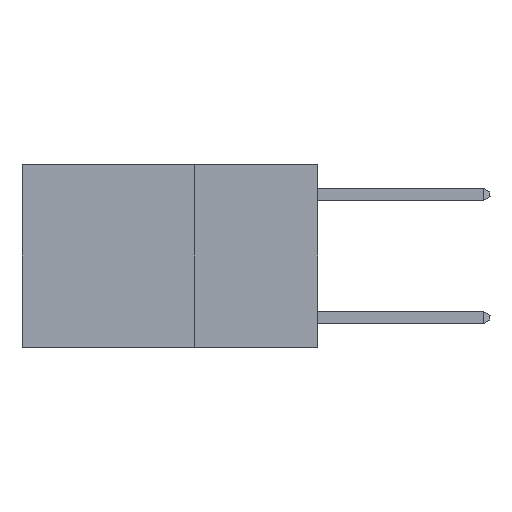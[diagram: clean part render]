
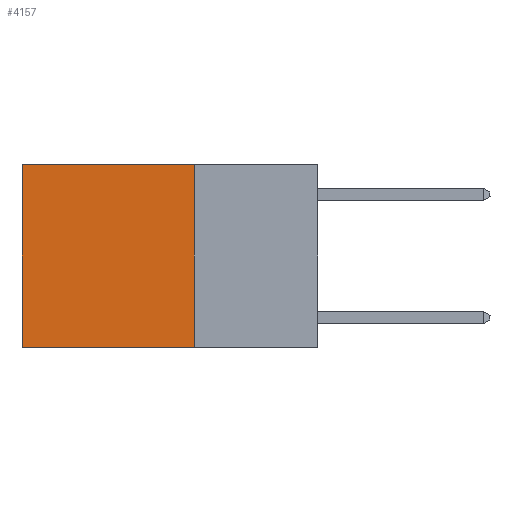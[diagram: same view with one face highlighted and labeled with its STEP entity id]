
A CAD part, left-side view. The second image highlights one B-rep face of the part: STEP entity #4157.
In plain terms, the highlighted planar face has unit normal (-1, 0, 0).
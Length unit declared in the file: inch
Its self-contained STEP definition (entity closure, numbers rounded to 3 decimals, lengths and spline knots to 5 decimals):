
#959 = VECTOR ( 'NONE', #4185, 39.37008 ) ;
#1105 = DIRECTION ( 'NONE',  ( 0., 0., -1. ) ) ;
#1452 = VECTOR ( 'NONE', #5163, 39.37008 ) ;
#1995 = EDGE_LOOP ( 'NONE', ( #10030, #11990, #5094, #4405 ) ) ;
#2158 = DIRECTION ( 'NONE',  ( 1., 0., 0. ) ) ;
#2170 = EDGE_CURVE ( 'NONE', #8054, #10831, #4980, .T. ) ;
#3110 = VECTOR ( 'NONE', #1105, 39.37008 ) ;
#3152 = PLANE ( 'NONE',  #8724 ) ;
#3427 = CARTESIAN_POINT ( 'NONE',  ( 0.2625, 0.25, -0.37 ) ) ;
#3644 = LINE ( 'NONE', #10941, #8235 ) ;
#3904 = EDGE_CURVE ( 'NONE', #10700, #11582, #8174, .T. ) ;
#4157 = ADVANCED_FACE ( 'NONE', ( #7967 ), #3152, .F. ) ;
#4185 = DIRECTION ( 'NONE',  ( 0., 1., 0. ) ) ;
#4405 = ORIENTED_EDGE ( 'NONE', *, *, #7796, .T. ) ;
#4980 = LINE ( 'NONE', #9995, #3110 ) ;
#5032 = CARTESIAN_POINT ( 'NONE',  ( 0.2625, 0.6, 0. ) ) ;
#5094 = ORIENTED_EDGE ( 'NONE', *, *, #2170, .F. ) ;
#5163 = DIRECTION ( 'NONE',  ( 0., 0., -1. ) ) ;
#5416 = EDGE_CURVE ( 'NONE', #10831, #11582, #3644, .T. ) ;
#6085 = LINE ( 'NONE', #7296, #959 ) ;
#6086 = CARTESIAN_POINT ( 'NONE',  ( 0.2625, 0.6, -0.37 ) ) ;
#7250 = DIRECTION ( 'NONE',  ( 0., 0., -1. ) ) ;
#7296 = CARTESIAN_POINT ( 'NONE',  ( 0.2625, 0.25, 0. ) ) ;
#7796 = EDGE_CURVE ( 'NONE', #8054, #10700, #6085, .T. ) ;
#7800 = CARTESIAN_POINT ( 'NONE',  ( 0.2625, 0.25, 0. ) ) ;
#7967 = FACE_OUTER_BOUND ( 'NONE', #1995, .T. ) ;
#8054 = VERTEX_POINT ( 'NONE', #7800 ) ;
#8174 = LINE ( 'NONE', #5032, #1452 ) ;
#8235 = VECTOR ( 'NONE', #10482, 39.37008 ) ;
#8724 = AXIS2_PLACEMENT_3D ( 'NONE', #12102, #2158, #7250 ) ;
#9995 = CARTESIAN_POINT ( 'NONE',  ( 0.2625, 0.25, 0. ) ) ;
#10030 = ORIENTED_EDGE ( 'NONE', *, *, #3904, .T. ) ;
#10482 = DIRECTION ( 'NONE',  ( 0., 1., 0. ) ) ;
#10700 = VERTEX_POINT ( 'NONE', #12173 ) ;
#10831 = VERTEX_POINT ( 'NONE', #3427 ) ;
#10941 = CARTESIAN_POINT ( 'NONE',  ( 0.2625, 0.25, -0.37 ) ) ;
#11582 = VERTEX_POINT ( 'NONE', #6086 ) ;
#11990 = ORIENTED_EDGE ( 'NONE', *, *, #5416, .F. ) ;
#12102 = CARTESIAN_POINT ( 'NONE',  ( 0.2625, 0.25, 0. ) ) ;
#12173 = CARTESIAN_POINT ( 'NONE',  ( 0.2625, 0.6, 0. ) ) ;
